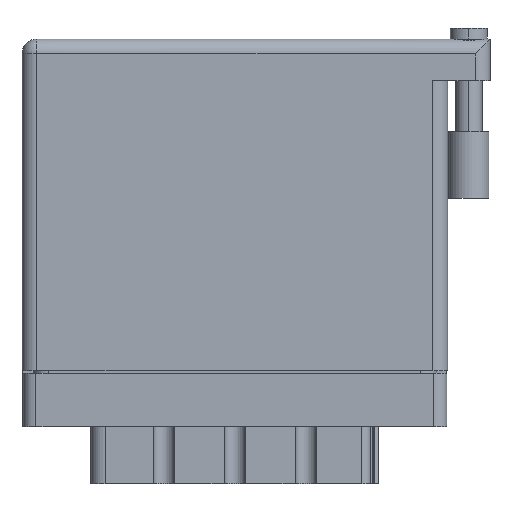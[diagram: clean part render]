
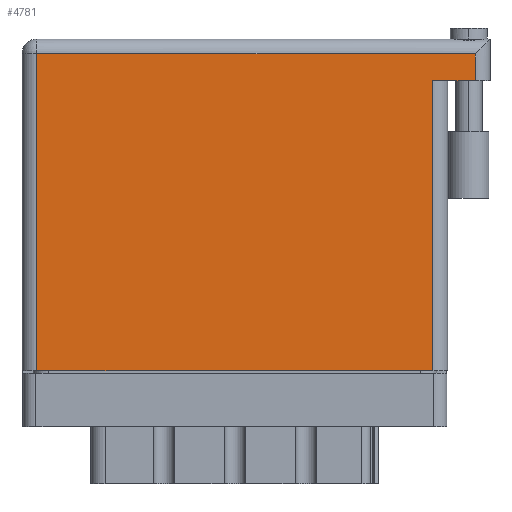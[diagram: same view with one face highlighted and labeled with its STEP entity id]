
A CAD part, front view. The second image highlights one B-rep face of the part: STEP entity #4781.
In plain terms, the highlighted face is planar.
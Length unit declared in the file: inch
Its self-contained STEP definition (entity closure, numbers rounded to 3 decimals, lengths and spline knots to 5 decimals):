
#1830 = LINE ( 'NONE', #15302, #27681 ) ;
#2287 = AXIS2_PLACEMENT_3D ( 'NONE', #7110, #26876, #27248 ) ;
#2406 = ORIENTED_EDGE ( 'NONE', *, *, #31849, .T. ) ;
#4781 = ADVANCED_FACE ( 'NONE', ( #35301 ), #18643, .F. ) ;
#5281 = VERTEX_POINT ( 'NONE', #10104 ) ;
#5646 = EDGE_CURVE ( 'NONE', #5281, #20744, #1830, .T. ) ;
#6592 = CARTESIAN_POINT ( 'NONE',  ( 0.07, 0., 0. ) ) ;
#6833 = DIRECTION ( 'NONE',  ( 0., -1., 0. ) ) ;
#7027 = EDGE_CURVE ( 'NONE', #12308, #16156, #28355, .T. ) ;
#7110 = CARTESIAN_POINT ( 'NONE',  ( 0., 1.566, 0. ) ) ;
#10011 = CARTESIAN_POINT ( 'NONE',  ( 1.938, 1.369, 0. ) ) ;
#10104 = CARTESIAN_POINT ( 'NONE',  ( 2.138, 1.369, 0. ) ) ;
#11817 = EDGE_CURVE ( 'NONE', #16156, #20744, #27935, .T. ) ;
#12153 = EDGE_CURVE ( 'NONE', #5281, #25615, #27659, .T. ) ;
#12308 = VERTEX_POINT ( 'NONE', #26796 ) ;
#14153 = ORIENTED_EDGE ( 'NONE', *, *, #11817, .T. ) ;
#14723 = EDGE_CURVE ( 'NONE', #25615, #19352, #26980, .T. ) ;
#15302 = CARTESIAN_POINT ( 'NONE',  ( 2.208, 1.369, 0. ) ) ;
#15910 = VECTOR ( 'NONE', #18780, 39.37008 ) ;
#16156 = VERTEX_POINT ( 'NONE', #33606 ) ;
#16184 = LINE ( 'NONE', #6592, #33974 ) ;
#18342 = CARTESIAN_POINT ( 'NONE',  ( 1.938, 1.369, 0. ) ) ;
#18643 = PLANE ( 'NONE',  #2287 ) ;
#18718 = DIRECTION ( 'NONE',  ( 0., 1., 0. ) ) ;
#18780 = DIRECTION ( 'NONE',  ( 1., 0., 0. ) ) ;
#19348 = CARTESIAN_POINT ( 'NONE',  ( 0., 1.496, 0. ) ) ;
#19352 = VERTEX_POINT ( 'NONE', #29521 ) ;
#20458 = DIRECTION ( 'NONE',  ( 0., 1., 0. ) ) ;
#20744 = VERTEX_POINT ( 'NONE', #10011 ) ;
#22989 = ORIENTED_EDGE ( 'NONE', *, *, #5646, .F. ) ;
#23174 = VECTOR ( 'NONE', #20458, 39.37008 ) ;
#23530 = DIRECTION ( 'NONE',  ( -1., 0., 0. ) ) ;
#23798 = CARTESIAN_POINT ( 'NONE',  ( 2.138, 1.566, 0. ) ) ;
#25615 = VERTEX_POINT ( 'NONE', #29619 ) ;
#25637 = VECTOR ( 'NONE', #30420, 39.37008 ) ;
#26796 = CARTESIAN_POINT ( 'NONE',  ( 0.07, 0., 0. ) ) ;
#26876 = DIRECTION ( 'NONE',  ( 0., 0., -1. ) ) ;
#26980 = LINE ( 'NONE', #19348, #25637 ) ;
#27010 = VECTOR ( 'NONE', #18718, 39.37008 ) ;
#27248 = DIRECTION ( 'NONE',  ( -1., 0., 0. ) ) ;
#27357 = ORIENTED_EDGE ( 'NONE', *, *, #14723, .T. ) ;
#27659 = LINE ( 'NONE', #23798, #23174 ) ;
#27681 = VECTOR ( 'NONE', #23530, 39.37008 ) ;
#27935 = LINE ( 'NONE', #18342, #27010 ) ;
#28355 = LINE ( 'NONE', #29979, #15910 ) ;
#29521 = CARTESIAN_POINT ( 'NONE',  ( 0.07, 1.496, 0. ) ) ;
#29619 = CARTESIAN_POINT ( 'NONE',  ( 2.138, 1.496, 0. ) ) ;
#29979 = CARTESIAN_POINT ( 'NONE',  ( 0., 0., 0. ) ) ;
#30420 = DIRECTION ( 'NONE',  ( -1., 0., 0. ) ) ;
#31049 = ORIENTED_EDGE ( 'NONE', *, *, #12153, .T. ) ;
#31849 = EDGE_CURVE ( 'NONE', #19352, #12308, #16184, .T. ) ;
#33606 = CARTESIAN_POINT ( 'NONE',  ( 1.938, 0., 0. ) ) ;
#33682 = EDGE_LOOP ( 'NONE', ( #35473, #14153, #22989, #31049, #27357, #2406 ) ) ;
#33974 = VECTOR ( 'NONE', #6833, 39.37008 ) ;
#35301 = FACE_OUTER_BOUND ( 'NONE', #33682, .T. ) ;
#35473 = ORIENTED_EDGE ( 'NONE', *, *, #7027, .T. ) ;
